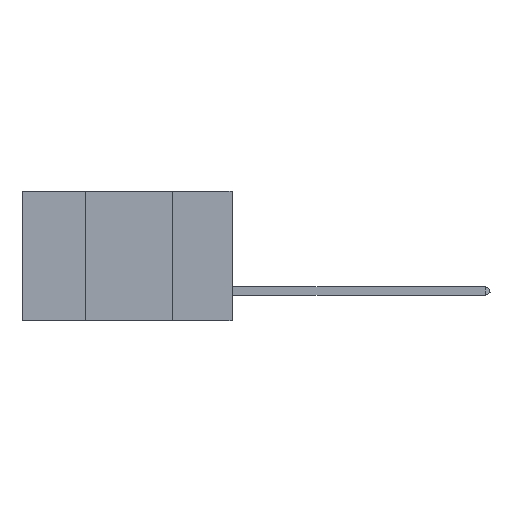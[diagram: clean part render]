
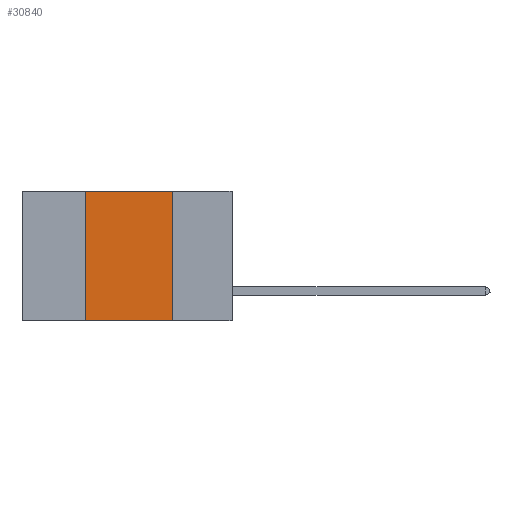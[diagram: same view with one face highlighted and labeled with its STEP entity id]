
A CAD part, left-side view. The second image highlights one B-rep face of the part: STEP entity #30840.
In plain terms, the highlighted planar face has unit normal (-1, 0, 0).
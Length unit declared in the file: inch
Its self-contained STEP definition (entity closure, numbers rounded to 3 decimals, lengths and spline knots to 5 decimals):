
#125 = VERTEX_POINT ( 'NONE', #20318 ) ;
#1776 = DIRECTION ( 'NONE',  ( 1., 0., 0. ) ) ;
#2918 = ORIENTED_EDGE ( 'NONE', *, *, #14780, .F. ) ;
#5155 = CARTESIAN_POINT ( 'NONE',  ( 0., 0.17, 0. ) ) ;
#5702 = DIRECTION ( 'NONE',  ( 0., 0., 1. ) ) ;
#5817 = DIRECTION ( 'NONE',  ( 0., 0., -1. ) ) ;
#6176 = FACE_OUTER_BOUND ( 'NONE', #26303, .T. ) ;
#6704 = LINE ( 'NONE', #47274, #36898 ) ;
#8467 = ORIENTED_EDGE ( 'NONE', *, *, #31377, .F. ) ;
#9667 = VERTEX_POINT ( 'NONE', #37053 ) ;
#10054 = DIRECTION ( 'NONE',  ( 0., 0., -1. ) ) ;
#11928 = CARTESIAN_POINT ( 'NONE',  ( 0., 0.17, 0. ) ) ;
#14780 = EDGE_CURVE ( 'NONE', #44302, #43605, #32858, .T. ) ;
#18260 = ORIENTED_EDGE ( 'NONE', *, *, #38385, .F. ) ;
#20318 = CARTESIAN_POINT ( 'NONE',  ( 0., 0.42, -0.37 ) ) ;
#24597 = DIRECTION ( 'NONE',  ( 0., -1., 0. ) ) ;
#26303 = EDGE_LOOP ( 'NONE', ( #2918, #18260, #8467, #32788 ) ) ;
#28716 = VECTOR ( 'NONE', #30101, 39.37008 ) ;
#28915 = CARTESIAN_POINT ( 'NONE',  ( 0., 0.6, 0. ) ) ;
#30101 = DIRECTION ( 'NONE',  ( 0., -1., 0. ) ) ;
#30840 = ADVANCED_FACE ( 'NONE', ( #6176 ), #39697, .F. ) ;
#31377 = EDGE_CURVE ( 'NONE', #125, #9667, #6704, .T. ) ;
#32788 = ORIENTED_EDGE ( 'NONE', *, *, #41170, .T. ) ;
#32858 = LINE ( 'NONE', #5155, #48269 ) ;
#33836 = CARTESIAN_POINT ( 'NONE',  ( 0., 0.17, -0.37 ) ) ;
#34064 = CARTESIAN_POINT ( 'NONE',  ( 0., 0.6, -0.37 ) ) ;
#36898 = VECTOR ( 'NONE', #5702, 39.37008 ) ;
#37053 = CARTESIAN_POINT ( 'NONE',  ( 0., 0.42, 0. ) ) ;
#38385 = EDGE_CURVE ( 'NONE', #9667, #44302, #45661, .T. ) ;
#38561 = AXIS2_PLACEMENT_3D ( 'NONE', #28915, #1776, #10054 ) ;
#39127 = VECTOR ( 'NONE', #24597, 39.37008 ) ;
#39697 = PLANE ( 'NONE',  #38561 ) ;
#41170 = EDGE_CURVE ( 'NONE', #125, #43605, #42935, .T. ) ;
#42935 = LINE ( 'NONE', #34064, #28716 ) ;
#43605 = VERTEX_POINT ( 'NONE', #33836 ) ;
#44302 = VERTEX_POINT ( 'NONE', #11928 ) ;
#45661 = LINE ( 'NONE', #47322, #39127 ) ;
#47274 = CARTESIAN_POINT ( 'NONE',  ( 0., 0.42, 0. ) ) ;
#47322 = CARTESIAN_POINT ( 'NONE',  ( 0., 0.6, 0. ) ) ;
#48269 = VECTOR ( 'NONE', #5817, 39.37008 ) ;
